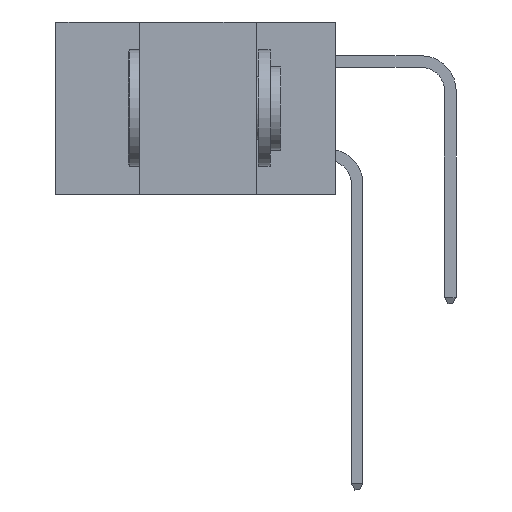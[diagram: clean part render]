
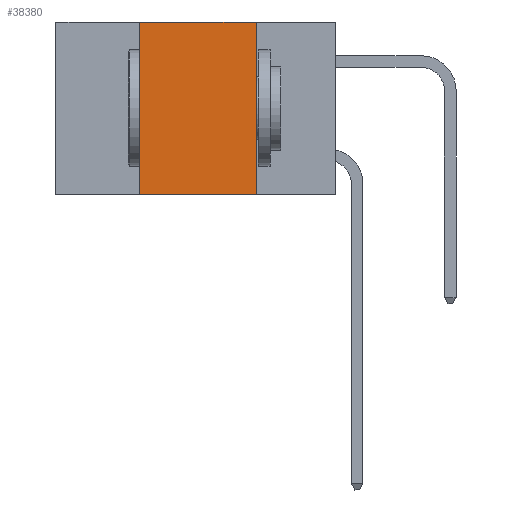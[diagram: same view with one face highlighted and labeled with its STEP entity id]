
A CAD part, left-side view. The second image highlights one B-rep face of the part: STEP entity #38380.
In plain terms, the highlighted planar face has unit normal (-1, 0, 0).
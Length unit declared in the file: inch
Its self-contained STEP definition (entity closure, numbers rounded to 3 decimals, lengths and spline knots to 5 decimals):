
#1959 = EDGE_CURVE ( 'NONE', #22630, #12429, #23409, .T. ) ;
#5018 = ORIENTED_EDGE ( 'NONE', *, *, #18556, .F. ) ;
#5785 = VECTOR ( 'NONE', #41046, 39.37008 ) ;
#8207 = ORIENTED_EDGE ( 'NONE', *, *, #1959, .F. ) ;
#8615 = VERTEX_POINT ( 'NONE', #17394 ) ;
#10154 = LINE ( 'NONE', #26915, #36388 ) ;
#10539 = LINE ( 'NONE', #19353, #16196 ) ;
#12429 = VERTEX_POINT ( 'NONE', #13085 ) ;
#13085 = CARTESIAN_POINT ( 'NONE',  ( 0., 0.17, 0. ) ) ;
#13476 = FACE_OUTER_BOUND ( 'NONE', #37686, .T. ) ;
#14939 = EDGE_CURVE ( 'NONE', #29644, #8615, #10539, .T. ) ;
#15020 = CARTESIAN_POINT ( 'NONE',  ( 0., 0.42, 0. ) ) ;
#15131 = CARTESIAN_POINT ( 'NONE',  ( 0., 0.42, -0.37 ) ) ;
#16196 = VECTOR ( 'NONE', #32477, 39.37008 ) ;
#16640 = AXIS2_PLACEMENT_3D ( 'NONE', #37895, #18383, #41316 ) ;
#17394 = CARTESIAN_POINT ( 'NONE',  ( 0., 0.17, -0.37 ) ) ;
#17951 = VECTOR ( 'NONE', #26583, 39.37008 ) ;
#18383 = DIRECTION ( 'NONE',  ( 1., 0., 0. ) ) ;
#18556 = EDGE_CURVE ( 'NONE', #29644, #22630, #25739, .T. ) ;
#19353 = CARTESIAN_POINT ( 'NONE',  ( 0., 0.6, -0.37 ) ) ;
#20419 = DIRECTION ( 'NONE',  ( 0., 0., -1. ) ) ;
#21472 = CARTESIAN_POINT ( 'NONE',  ( 0., 0.6, 0. ) ) ;
#22181 = EDGE_CURVE ( 'NONE', #12429, #8615, #10154, .T. ) ;
#22630 = VERTEX_POINT ( 'NONE', #15020 ) ;
#23409 = LINE ( 'NONE', #21472, #5785 ) ;
#25739 = LINE ( 'NONE', #29908, #17951 ) ;
#26583 = DIRECTION ( 'NONE',  ( 0., 0., 1. ) ) ;
#26915 = CARTESIAN_POINT ( 'NONE',  ( 0., 0.17, 0. ) ) ;
#28237 = PLANE ( 'NONE',  #16640 ) ;
#29644 = VERTEX_POINT ( 'NONE', #15131 ) ;
#29908 = CARTESIAN_POINT ( 'NONE',  ( 0., 0.42, 0. ) ) ;
#32477 = DIRECTION ( 'NONE',  ( 0., -1., 0. ) ) ;
#35473 = ORIENTED_EDGE ( 'NONE', *, *, #14939, .T. ) ;
#36388 = VECTOR ( 'NONE', #20419, 39.37008 ) ;
#37686 = EDGE_LOOP ( 'NONE', ( #39064, #8207, #5018, #35473 ) ) ;
#37895 = CARTESIAN_POINT ( 'NONE',  ( 0., 0.6, 0. ) ) ;
#38380 = ADVANCED_FACE ( 'NONE', ( #13476 ), #28237, .F. ) ;
#39064 = ORIENTED_EDGE ( 'NONE', *, *, #22181, .F. ) ;
#41046 = DIRECTION ( 'NONE',  ( 0., -1., 0. ) ) ;
#41316 = DIRECTION ( 'NONE',  ( 0., 0., -1. ) ) ;
